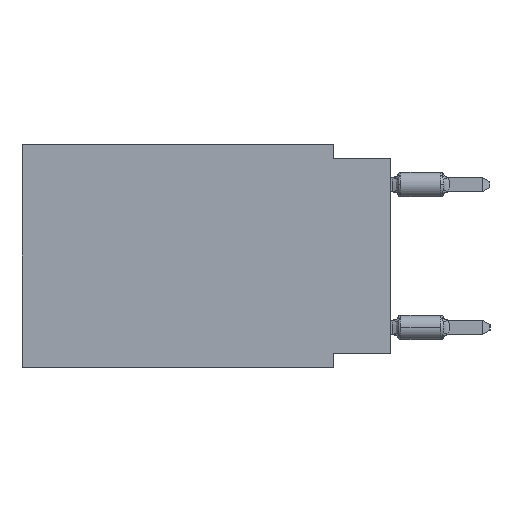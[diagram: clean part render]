
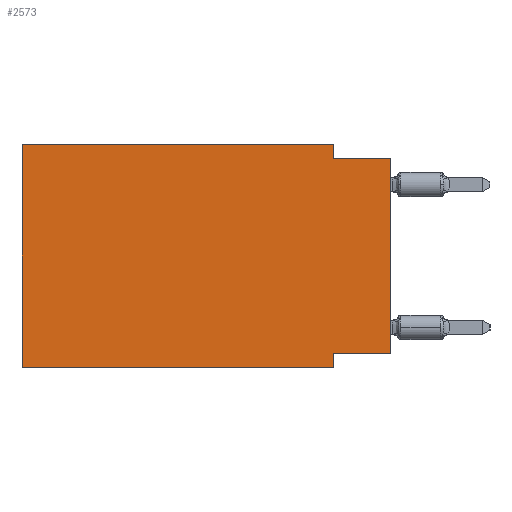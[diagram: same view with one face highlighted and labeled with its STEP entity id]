
A CAD part, left-side view. The second image highlights one B-rep face of the part: STEP entity #2573.
In plain terms, the highlighted planar face has unit normal (-1, 0, 0).
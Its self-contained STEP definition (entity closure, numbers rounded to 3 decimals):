
#281 = EDGE_LOOP ( 'NONE', ( #20327, #12931, #12451, #2540, #12240, #3802, #5244, #24367 ) ) ;
#705 = CARTESIAN_POINT ( 'NONE',  ( 0., 16.383, 0. ) ) ;
#2380 = FACE_OUTER_BOUND ( 'NONE', #281, .T. ) ;
#2540 = ORIENTED_EDGE ( 'NONE', *, *, #13610, .F. ) ;
#2573 = ADVANCED_FACE ( 'NONE', ( #2380 ), #8722, .F. ) ;
#2761 = LINE ( 'NONE', #10671, #7701 ) ;
#2801 = CARTESIAN_POINT ( 'NONE',  ( 0., 16.383, -9.906 ) ) ;
#2923 = LINE ( 'NONE', #4865, #21851 ) ;
#3137 = DIRECTION ( 'NONE',  ( 0., -1., 0. ) ) ;
#3721 = CARTESIAN_POINT ( 'NONE',  ( 0., 0., -0.635 ) ) ;
#3802 = ORIENTED_EDGE ( 'NONE', *, *, #19058, .T. ) ;
#4103 = VERTEX_POINT ( 'NONE', #5861 ) ;
#4124 = EDGE_CURVE ( 'NONE', #6314, #21648, #23743, .T. ) ;
#4865 = CARTESIAN_POINT ( 'NONE',  ( 0., 0., -9.271 ) ) ;
#5077 = DIRECTION ( 'NONE',  ( 0., 0., 1. ) ) ;
#5244 = ORIENTED_EDGE ( 'NONE', *, *, #4124, .F. ) ;
#5861 = CARTESIAN_POINT ( 'NONE',  ( 0., 2.54, 0. ) ) ;
#6314 = VERTEX_POINT ( 'NONE', #10584 ) ;
#6431 = DIRECTION ( 'NONE',  ( 0., 0., -1. ) ) ;
#6435 = AXIS2_PLACEMENT_3D ( 'NONE', #705, #8585, #8220 ) ;
#6514 = EDGE_CURVE ( 'NONE', #21558, #11004, #13327, .T. ) ;
#6554 = CARTESIAN_POINT ( 'NONE',  ( 0., 16.383, 0. ) ) ;
#6900 = LINE ( 'NONE', #12986, #18608 ) ;
#7213 = DIRECTION ( 'NONE',  ( 0., 1., 0. ) ) ;
#7701 = VECTOR ( 'NONE', #18590, 1000. ) ;
#7716 = CARTESIAN_POINT ( 'NONE',  ( 0., 16.383, 0. ) ) ;
#8220 = DIRECTION ( 'NONE',  ( 0., 0., -1. ) ) ;
#8312 = EDGE_CURVE ( 'NONE', #10556, #12289, #6900, .T. ) ;
#8585 = DIRECTION ( 'NONE',  ( 1., 0., 0. ) ) ;
#8722 = PLANE ( 'NONE',  #6435 ) ;
#9040 = CARTESIAN_POINT ( 'NONE',  ( 0., 16.383, 0. ) ) ;
#9427 = CARTESIAN_POINT ( 'NONE',  ( 0., 2.54, -9.906 ) ) ;
#10203 = DIRECTION ( 'NONE',  ( 0., -1., 0. ) ) ;
#10342 = CARTESIAN_POINT ( 'NONE',  ( 0., 2.54, -0.635 ) ) ;
#10445 = LINE ( 'NONE', #6554, #17617 ) ;
#10556 = VERTEX_POINT ( 'NONE', #10878 ) ;
#10584 = CARTESIAN_POINT ( 'NONE',  ( 0., 2.54, -9.271 ) ) ;
#10594 = VECTOR ( 'NONE', #3137, 1000. ) ;
#10671 = CARTESIAN_POINT ( 'NONE',  ( 0., 16.383, -9.906 ) ) ;
#10878 = CARTESIAN_POINT ( 'NONE',  ( 0., 0., -9.271 ) ) ;
#11004 = VERTEX_POINT ( 'NONE', #7716 ) ;
#11239 = DIRECTION ( 'NONE',  ( 0., 0., 1. ) ) ;
#11311 = LINE ( 'NONE', #20907, #10594 ) ;
#12111 = VECTOR ( 'NONE', #17926, 1000. ) ;
#12240 = ORIENTED_EDGE ( 'NONE', *, *, #6514, .F. ) ;
#12289 = VERTEX_POINT ( 'NONE', #3721 ) ;
#12451 = ORIENTED_EDGE ( 'NONE', *, *, #23800, .F. ) ;
#12546 = EDGE_CURVE ( 'NONE', #16284, #12289, #11311, .T. ) ;
#12931 = ORIENTED_EDGE ( 'NONE', *, *, #12546, .F. ) ;
#12986 = CARTESIAN_POINT ( 'NONE',  ( 0., 0., 0. ) ) ;
#13327 = LINE ( 'NONE', #9040, #17035 ) ;
#13610 = EDGE_CURVE ( 'NONE', #11004, #4103, #10445, .T. ) ;
#16284 = VERTEX_POINT ( 'NONE', #10342 ) ;
#17035 = VECTOR ( 'NONE', #11239, 1000. ) ;
#17617 = VECTOR ( 'NONE', #10203, 1000. ) ;
#17926 = DIRECTION ( 'NONE',  ( 0., 0., -1. ) ) ;
#18590 = DIRECTION ( 'NONE',  ( 0., -1., 0. ) ) ;
#18608 = VECTOR ( 'NONE', #5077, 1000. ) ;
#19058 = EDGE_CURVE ( 'NONE', #21558, #21648, #2761, .T. ) ;
#19733 = CARTESIAN_POINT ( 'NONE',  ( 0., 2.54, -9.906 ) ) ;
#19794 = VECTOR ( 'NONE', #6431, 1000. ) ;
#20327 = ORIENTED_EDGE ( 'NONE', *, *, #8312, .T. ) ;
#20907 = CARTESIAN_POINT ( 'NONE',  ( 0., 0., -0.635 ) ) ;
#21558 = VERTEX_POINT ( 'NONE', #2801 ) ;
#21648 = VERTEX_POINT ( 'NONE', #9427 ) ;
#21851 = VECTOR ( 'NONE', #7213, 1000. ) ;
#22121 = LINE ( 'NONE', #24177, #19794 ) ;
#23743 = LINE ( 'NONE', #19733, #12111 ) ;
#23800 = EDGE_CURVE ( 'NONE', #4103, #16284, #22121, .T. ) ;
#23930 = EDGE_CURVE ( 'NONE', #10556, #6314, #2923, .T. ) ;
#24177 = CARTESIAN_POINT ( 'NONE',  ( 0., 2.54, 0. ) ) ;
#24367 = ORIENTED_EDGE ( 'NONE', *, *, #23930, .F. ) ;
